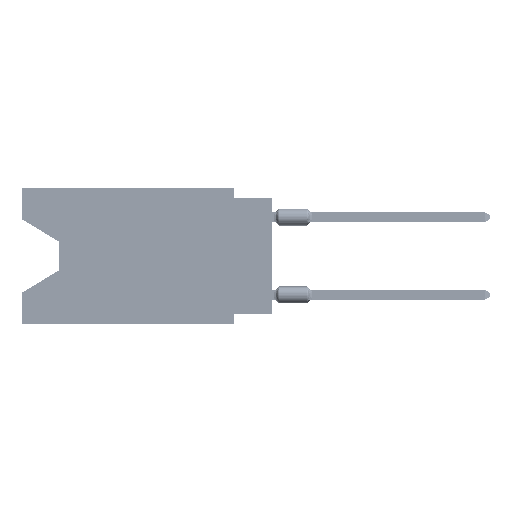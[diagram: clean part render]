
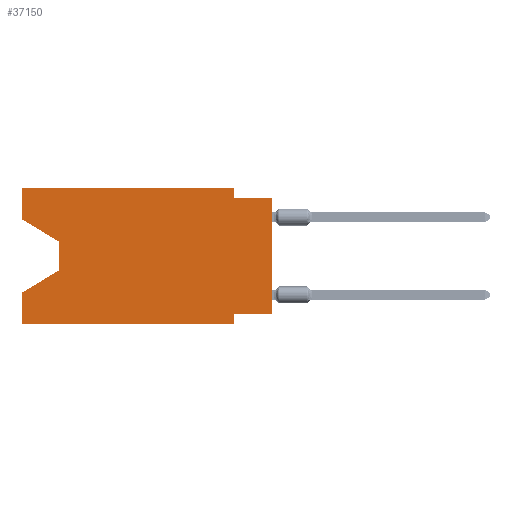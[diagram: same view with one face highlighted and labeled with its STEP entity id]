
A CAD part, left-side view. The second image highlights one B-rep face of the part: STEP entity #37150.
In plain terms, the highlighted planar face has unit normal (-1, 0, 0).
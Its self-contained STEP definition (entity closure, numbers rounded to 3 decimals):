
#828 = CARTESIAN_POINT ( 'NONE',  ( 0., 16.383, -6.852 ) ) ;
#960 = CARTESIAN_POINT ( 'NONE',  ( 0., 2.54, -8.89 ) ) ;
#1204 = VECTOR ( 'NONE', #16699, 1000. ) ;
#2589 = VECTOR ( 'NONE', #3858, 1000. ) ;
#2835 = ORIENTED_EDGE ( 'NONE', *, *, #32799, .F. ) ;
#2907 = VECTOR ( 'NONE', #11010, 1000. ) ;
#3146 = DIRECTION ( 'NONE',  ( 0., 0., 1. ) ) ;
#3307 = VECTOR ( 'NONE', #49758, 1000. ) ;
#3694 = FACE_OUTER_BOUND ( 'NONE', #64591, .T. ) ;
#3858 = DIRECTION ( 'NONE',  ( 0., 0., -1. ) ) ;
#4046 = DIRECTION ( 'NONE',  ( 0., -1., 0. ) ) ;
#4381 = VERTEX_POINT ( 'NONE', #58855 ) ;
#4875 = VECTOR ( 'NONE', #4046, 1000. ) ;
#5330 = CARTESIAN_POINT ( 'NONE',  ( 0., 16.383, 0. ) ) ;
#6325 = DIRECTION ( 'NONE',  ( 0., 0., -1. ) ) ;
#6900 = CARTESIAN_POINT ( 'NONE',  ( 0., 13.97, -5.385 ) ) ;
#7648 = CARTESIAN_POINT ( 'NONE',  ( 0., 16.383, -2.038 ) ) ;
#7692 = EDGE_CURVE ( 'NONE', #55957, #29563, #35589, .T. ) ;
#7700 = CARTESIAN_POINT ( 'NONE',  ( 0., 13.97, -5.385 ) ) ;
#9383 = LINE ( 'NONE', #64882, #4875 ) ;
#9782 = VERTEX_POINT ( 'NONE', #37337 ) ;
#11010 = DIRECTION ( 'NONE',  ( 0., -1., 0. ) ) ;
#16699 = DIRECTION ( 'NONE',  ( 0., -0.855, -0.519 ) ) ;
#16737 = CARTESIAN_POINT ( 'NONE',  ( 0., 2.54, 0. ) ) ;
#17766 = CARTESIAN_POINT ( 'NONE',  ( 0., 0., 0. ) ) ;
#19374 = CARTESIAN_POINT ( 'NONE',  ( 0., 13.97, -3.505 ) ) ;
#20486 = ORIENTED_EDGE ( 'NONE', *, *, #7692, .T. ) ;
#20762 = DIRECTION ( 'NONE',  ( 0., 0., 1. ) ) ;
#21053 = DIRECTION ( 'NONE',  ( 1., 0., 0. ) ) ;
#21534 = ORIENTED_EDGE ( 'NONE', *, *, #52572, .F. ) ;
#22126 = ORIENTED_EDGE ( 'NONE', *, *, #30600, .F. ) ;
#22482 = LINE ( 'NONE', #17766, #51054 ) ;
#23124 = CARTESIAN_POINT ( 'NONE',  ( 0., 16.383, -8.89 ) ) ;
#23371 = VECTOR ( 'NONE', #25595, 1000. ) ;
#23479 = DIRECTION ( 'NONE',  ( 0., 0., 1. ) ) ;
#23543 = CARTESIAN_POINT ( 'NONE',  ( 0., 16.383, 0. ) ) ;
#23558 = CARTESIAN_POINT ( 'NONE',  ( 0., 2.54, -8.89 ) ) ;
#24101 = PLANE ( 'NONE',  #27248 ) ;
#25595 = DIRECTION ( 'NONE',  ( 0., 0., -1. ) ) ;
#25772 = EDGE_CURVE ( 'NONE', #35752, #9782, #30807, .T. ) ;
#26654 = DIRECTION ( 'NONE',  ( 0., -1., 0. ) ) ;
#27248 = AXIS2_PLACEMENT_3D ( 'NONE', #5330, #21053, #6325 ) ;
#27470 = EDGE_CURVE ( 'NONE', #29563, #38400, #27792, .T. ) ;
#27660 = LINE ( 'NONE', #53029, #2907 ) ;
#27792 = LINE ( 'NONE', #7700, #29713 ) ;
#28232 = EDGE_CURVE ( 'NONE', #36419, #57641, #51637, .T. ) ;
#28527 = ORIENTED_EDGE ( 'NONE', *, *, #25772, .F. ) ;
#28727 = ORIENTED_EDGE ( 'NONE', *, *, #38338, .T. ) ;
#28784 = CARTESIAN_POINT ( 'NONE',  ( 0., 16.383, -2.038 ) ) ;
#28820 = VECTOR ( 'NONE', #49941, 1000. ) ;
#29563 = VERTEX_POINT ( 'NONE', #6900 ) ;
#29713 = VECTOR ( 'NONE', #53177, 1000. ) ;
#30260 = CARTESIAN_POINT ( 'NONE',  ( 0., 13.97, -3.505 ) ) ;
#30600 = EDGE_CURVE ( 'NONE', #56764, #38400, #43250, .T. ) ;
#30807 = LINE ( 'NONE', #56839, #45013 ) ;
#32730 = EDGE_CURVE ( 'NONE', #35752, #55957, #57805, .T. ) ;
#32799 = EDGE_CURVE ( 'NONE', #59992, #4381, #39736, .T. ) ;
#34774 = VERTEX_POINT ( 'NONE', #37376 ) ;
#35589 = LINE ( 'NONE', #30260, #2589 ) ;
#35752 = VERTEX_POINT ( 'NONE', #28784 ) ;
#36419 = VERTEX_POINT ( 'NONE', #16737 ) ;
#37150 = ADVANCED_FACE ( 'NONE', ( #3694 ), #24101, .F. ) ;
#37337 = CARTESIAN_POINT ( 'NONE',  ( 0., 16.383, 0. ) ) ;
#37376 = CARTESIAN_POINT ( 'NONE',  ( 0., 0., -0.635 ) ) ;
#38338 = EDGE_CURVE ( 'NONE', #56764, #38984, #9383, .T. ) ;
#38400 = VERTEX_POINT ( 'NONE', #828 ) ;
#38652 = VECTOR ( 'NONE', #26654, 1000. ) ;
#38984 = VERTEX_POINT ( 'NONE', #960 ) ;
#39736 = LINE ( 'NONE', #49415, #3307 ) ;
#43250 = LINE ( 'NONE', #23543, #66109 ) ;
#44924 = LINE ( 'NONE', #23558, #28820 ) ;
#45013 = VECTOR ( 'NONE', #20762, 1000. ) ;
#45070 = ORIENTED_EDGE ( 'NONE', *, *, #56987, .F. ) ;
#46298 = CARTESIAN_POINT ( 'NONE',  ( 0., 2.54, 0. ) ) ;
#47128 = ORIENTED_EDGE ( 'NONE', *, *, #57973, .T. ) ;
#47335 = CARTESIAN_POINT ( 'NONE',  ( 0., 16.383, 0. ) ) ;
#47355 = ORIENTED_EDGE ( 'NONE', *, *, #32730, .T. ) ;
#49030 = CARTESIAN_POINT ( 'NONE',  ( 0., 0., -8.255 ) ) ;
#49415 = CARTESIAN_POINT ( 'NONE',  ( 0., 0., -8.255 ) ) ;
#49758 = DIRECTION ( 'NONE',  ( 0., 1., 0. ) ) ;
#49941 = DIRECTION ( 'NONE',  ( 0., 0., -1. ) ) ;
#51054 = VECTOR ( 'NONE', #23479, 1000. ) ;
#51637 = LINE ( 'NONE', #46298, #23371 ) ;
#51695 = LINE ( 'NONE', #47335, #38652 ) ;
#52572 = EDGE_CURVE ( 'NONE', #4381, #38984, #44924, .T. ) ;
#53029 = CARTESIAN_POINT ( 'NONE',  ( 0., 0., -0.635 ) ) ;
#53177 = DIRECTION ( 'NONE',  ( 0., 0.855, -0.519 ) ) ;
#55957 = VERTEX_POINT ( 'NONE', #19374 ) ;
#56764 = VERTEX_POINT ( 'NONE', #23124 ) ;
#56839 = CARTESIAN_POINT ( 'NONE',  ( 0., 16.383, 0. ) ) ;
#56987 = EDGE_CURVE ( 'NONE', #57641, #34774, #27660, .T. ) ;
#57374 = ORIENTED_EDGE ( 'NONE', *, *, #28232, .F. ) ;
#57512 = ORIENTED_EDGE ( 'NONE', *, *, #65409, .F. ) ;
#57641 = VERTEX_POINT ( 'NONE', #59272 ) ;
#57805 = LINE ( 'NONE', #7648, #1204 ) ;
#57973 = EDGE_CURVE ( 'NONE', #59992, #34774, #22482, .T. ) ;
#58855 = CARTESIAN_POINT ( 'NONE',  ( 0., 2.54, -8.255 ) ) ;
#59272 = CARTESIAN_POINT ( 'NONE',  ( 0., 2.54, -0.635 ) ) ;
#59992 = VERTEX_POINT ( 'NONE', #49030 ) ;
#64273 = ORIENTED_EDGE ( 'NONE', *, *, #27470, .T. ) ;
#64591 = EDGE_LOOP ( 'NONE', ( #47355, #20486, #64273, #22126, #28727, #21534, #2835, #47128, #45070, #57374, #57512, #28527 ) ) ;
#64882 = CARTESIAN_POINT ( 'NONE',  ( 0., 16.383, -8.89 ) ) ;
#65409 = EDGE_CURVE ( 'NONE', #9782, #36419, #51695, .T. ) ;
#66109 = VECTOR ( 'NONE', #3146, 1000. ) ;
